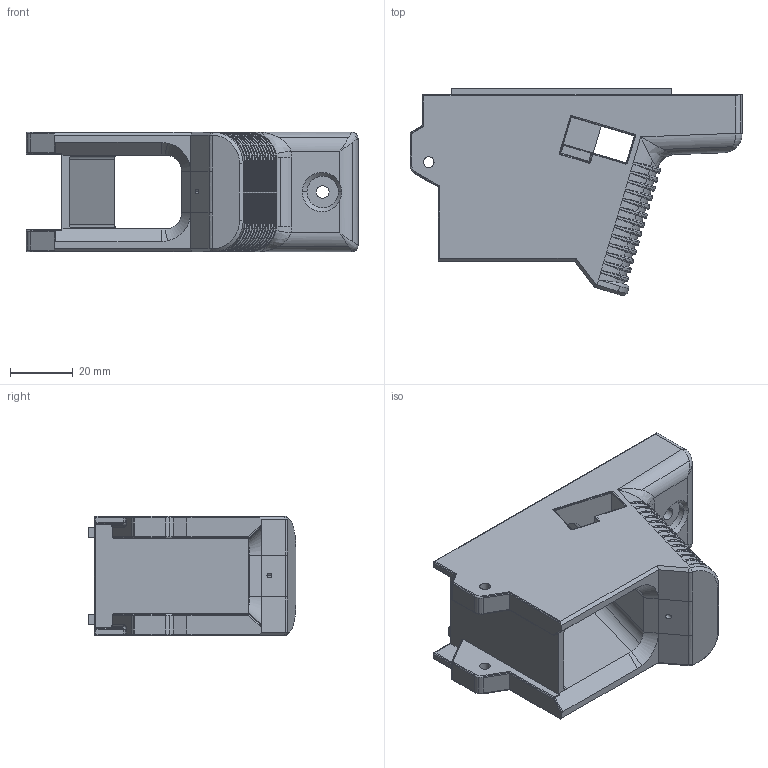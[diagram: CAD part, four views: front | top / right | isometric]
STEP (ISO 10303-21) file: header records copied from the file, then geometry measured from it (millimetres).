
FILE_DESCRIPTION(('STEP AP214'),'1');
FILE_NAME('MOD9_magwell grip IMA.stp','2020-07-20T11:35:56',(' '),(' '),'Spatial InterOp 3D',' ',' ');
FILE_SCHEMA(('AUTOMOTIVE_DESIGN { 1 0 10303 214 1 1 1 1 }'));
Length unit declared in the file: metre
Products named in the file (1): ASM Body
Bounding box: 105.51 x 66.04 x 38 mm (x, y, z)
Volume: 103766.6 mm3; surface area: 27857.4 mm2
Topology: 1 solids, 1 shells, 643 faces, 1677 edges, 1029 vertices
Faces by surface type: cylinder 342, plane 158, torus 73, bspline 56, sphere 12, cone 2
Entity records: 26431 total; most frequent: CARTESIAN_POINT 10913, ORIENTED_EDGE 3338, DIRECTION 3201, EDGE_CURVE 1669, AXIS2_PLACEMENT_3D 1224, VERTEX_POINT 1029, LINE 753, VECTOR 753
